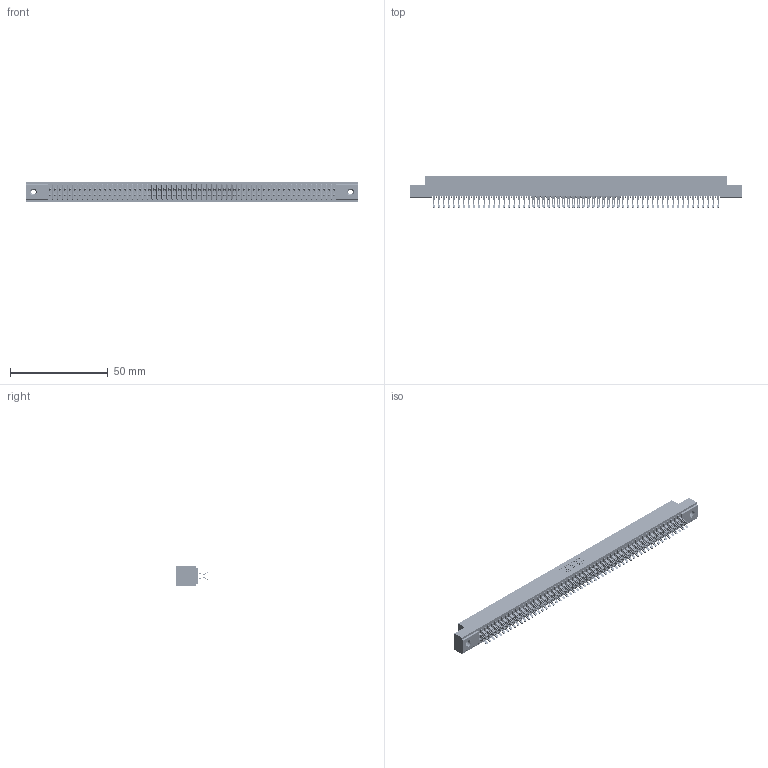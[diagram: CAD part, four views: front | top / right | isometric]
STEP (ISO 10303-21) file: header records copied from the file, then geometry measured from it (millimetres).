
FILE_DESCRIPTION (( 'STEP AP203' ), '1' );
FILE_NAME ('391-116-555-207.STEP', '2018-08-09T23:19:55', ( '' ), ( '' ), 'SwSTEP 2.0', 'SolidWorks 2016', '' );
FILE_SCHEMA (( 'CONFIG_CONTROL_DESIGN' ));
Length unit declared in the file: inch
Products named in the file (4): 391-116-555-207; 341 Part_.156 (3.96) Dia Mounting Holes; 341-292-001_341-292-155; 345-250-001_345-250-005-103
Assembly tree (119 placements, depth 2):
  391-116-555-207
    341 Part_.156 (3.96) Dia Mounting Holes
    341-292-001_341-292-155  x116
    345-250-001_345-250-005-103  x2
Bounding box: 169.54 x 16.31 x 10.16 mm (x, y, z)
Volume: 12668.1 mm3; surface area: 23974.5 mm2
Topology: 119 solids, 119 shells, 9224 faces, 27538 edges, 17922 vertices
Faces by surface type: plane 4972, cylinder 4004, sphere 118, torus 118, cone 12
Entity records: 69716 total; most frequent: CARTESIAN_POINT 11587, ORIENTED_EDGE 11500, DIRECTION 11234, EDGE_CURVE 5750, VECTOR 4644, LINE 4644, VERTEX_POINT 3632, AXIS2_PLACEMENT_3D 3295
